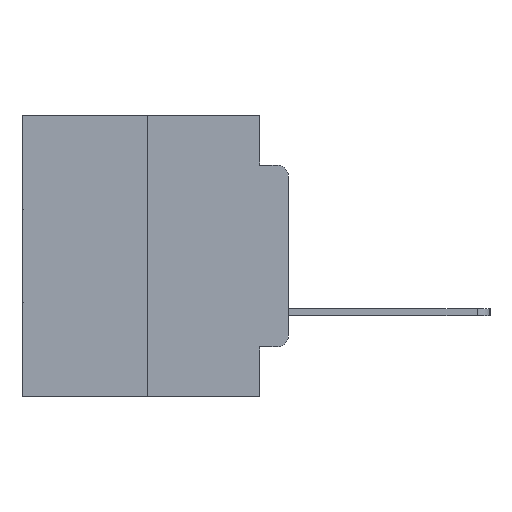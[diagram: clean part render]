
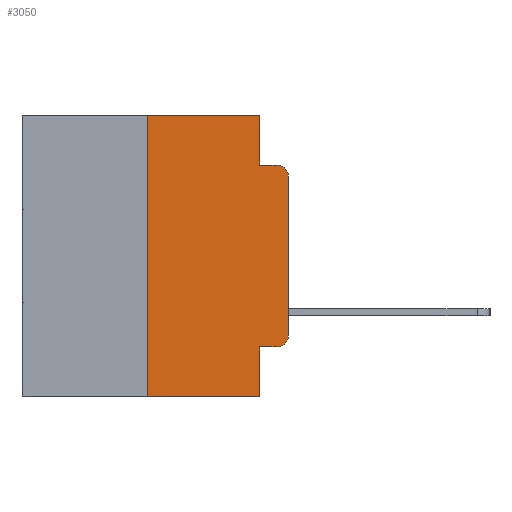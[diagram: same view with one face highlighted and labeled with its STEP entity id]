
A CAD part, left-side view. The second image highlights one B-rep face of the part: STEP entity #3050.
In plain terms, the highlighted planar face has unit normal (-1, 0, 0).
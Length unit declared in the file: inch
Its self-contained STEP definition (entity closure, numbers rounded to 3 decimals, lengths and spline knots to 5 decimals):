
#287 = LINE ( 'NONE', #20681, #16627 ) ;
#682 = VERTEX_POINT ( 'NONE', #21730 ) ;
#953 = VERTEX_POINT ( 'NONE', #15292 ) ;
#1065 = CARTESIAN_POINT ( 'NONE',  ( 0., 0.051, -0.0885 ) ) ;
#1193 = VECTOR ( 'NONE', #20912, 39.37008 ) ;
#1335 = VERTEX_POINT ( 'NONE', #1065 ) ;
#1770 = DIRECTION ( 'NONE',  ( -1., 0., 0. ) ) ;
#2549 = LINE ( 'NONE', #22921, #1193 ) ;
#3050 = ADVANCED_FACE ( 'NONE', ( #18681 ), #3953, .F. ) ;
#3126 = VERTEX_POINT ( 'NONE', #4517 ) ;
#3330 = ORIENTED_EDGE ( 'NONE', *, *, #9756, .F. ) ;
#3758 = CARTESIAN_POINT ( 'NONE',  ( 0., 0., -0.1085 ) ) ;
#3865 = CARTESIAN_POINT ( 'NONE',  ( 0., 0.473, -0.5 ) ) ;
#3953 = PLANE ( 'NONE',  #22412 ) ;
#4390 = VECTOR ( 'NONE', #15495, 39.37008 ) ;
#4517 = CARTESIAN_POINT ( 'NONE',  ( 0., 0.051, 0. ) ) ;
#4743 = CARTESIAN_POINT ( 'NONE',  ( 0., 0.051, -0.4115 ) ) ;
#4777 = AXIS2_PLACEMENT_3D ( 'NONE', #14542, #1770, #16639 ) ;
#5017 = CARTESIAN_POINT ( 'NONE',  ( 0., 0.051, -0.4115 ) ) ;
#5061 = CARTESIAN_POINT ( 'NONE',  ( 0., 0.051, 0. ) ) ;
#5077 = LINE ( 'NONE', #5017, #4390 ) ;
#5211 = VERTEX_POINT ( 'NONE', #20347 ) ;
#5696 = DIRECTION ( 'NONE',  ( 0., 0., 1. ) ) ;
#6668 = LINE ( 'NONE', #22225, #12323 ) ;
#6781 = CIRCLE ( 'NONE', #16351, 0.02 ) ;
#7011 = VERTEX_POINT ( 'NONE', #22452 ) ;
#7054 = EDGE_CURVE ( 'NONE', #9813, #682, #10407, .T. ) ;
#7096 = CARTESIAN_POINT ( 'NONE',  ( 0., 0.25, 0. ) ) ;
#7730 = ORIENTED_EDGE ( 'NONE', *, *, #14935, .T. ) ;
#7987 = EDGE_CURVE ( 'NONE', #26678, #3126, #14016, .T. ) ;
#8109 = CARTESIAN_POINT ( 'NONE',  ( 0., 0.473, 0. ) ) ;
#8330 = DIRECTION ( 'NONE',  ( 0., -1., 0. ) ) ;
#8448 = VECTOR ( 'NONE', #17324, 39.37008 ) ;
#8836 = VERTEX_POINT ( 'NONE', #9637 ) ;
#9637 = CARTESIAN_POINT ( 'NONE',  ( 0., 0.25, -0.5 ) ) ;
#9711 = VECTOR ( 'NONE', #12761, 39.37008 ) ;
#9756 = EDGE_CURVE ( 'NONE', #8836, #26678, #6668, .T. ) ;
#9813 = VERTEX_POINT ( 'NONE', #3758 ) ;
#9987 = EDGE_CURVE ( 'NONE', #23735, #7011, #2549, .T. ) ;
#10373 = LINE ( 'NONE', #14833, #9711 ) ;
#10398 = ORIENTED_EDGE ( 'NONE', *, *, #20171, .F. ) ;
#10407 = CIRCLE ( 'NONE', #4777, 0.02 ) ;
#10725 = EDGE_CURVE ( 'NONE', #3126, #1335, #20560, .T. ) ;
#11548 = DIRECTION ( 'NONE',  ( -1., 0., 0. ) ) ;
#12323 = VECTOR ( 'NONE', #5696, 39.37008 ) ;
#12624 = DIRECTION ( 'NONE',  ( 0., 0., -1. ) ) ;
#12761 = DIRECTION ( 'NONE',  ( 0., 0., 1. ) ) ;
#13661 = EDGE_CURVE ( 'NONE', #953, #5211, #6781, .T. ) ;
#14016 = LINE ( 'NONE', #15214, #8448 ) ;
#14495 = VECTOR ( 'NONE', #17643, 39.37008 ) ;
#14542 = CARTESIAN_POINT ( 'NONE',  ( 0., 0.02, -0.1085 ) ) ;
#14612 = ORIENTED_EDGE ( 'NONE', *, *, #7987, .F. ) ;
#14833 = CARTESIAN_POINT ( 'NONE',  ( 0., 0., 0. ) ) ;
#14935 = EDGE_CURVE ( 'NONE', #5211, #9813, #10373, .T. ) ;
#15214 = CARTESIAN_POINT ( 'NONE',  ( 0., 0.473, 0. ) ) ;
#15292 = CARTESIAN_POINT ( 'NONE',  ( 0., 0.02, -0.4115 ) ) ;
#15495 = DIRECTION ( 'NONE',  ( 0., -1., 0. ) ) ;
#15611 = ORIENTED_EDGE ( 'NONE', *, *, #13661, .T. ) ;
#16351 = AXIS2_PLACEMENT_3D ( 'NONE', #23712, #11548, #25697 ) ;
#16627 = VECTOR ( 'NONE', #8330, 39.37008 ) ;
#16639 = DIRECTION ( 'NONE',  ( 0., 0., -1. ) ) ;
#17220 = EDGE_CURVE ( 'NONE', #8836, #7011, #19909, .T. ) ;
#17324 = DIRECTION ( 'NONE',  ( 0., -1., 0. ) ) ;
#17643 = DIRECTION ( 'NONE',  ( 0., 0., -1. ) ) ;
#18681 = FACE_OUTER_BOUND ( 'NONE', #19276, .T. ) ;
#18788 = ORIENTED_EDGE ( 'NONE', *, *, #7054, .T. ) ;
#19276 = EDGE_LOOP ( 'NONE', ( #7730, #18788, #10398, #21920, #14612, #3330, #25946, #25743, #26275, #15611 ) ) ;
#19279 = VECTOR ( 'NONE', #20575, 39.37008 ) ;
#19909 = LINE ( 'NONE', #3865, #19279 ) ;
#20171 = EDGE_CURVE ( 'NONE', #1335, #682, #287, .T. ) ;
#20347 = CARTESIAN_POINT ( 'NONE',  ( 0., 0., -0.3915 ) ) ;
#20560 = LINE ( 'NONE', #5061, #14495 ) ;
#20575 = DIRECTION ( 'NONE',  ( 0., -1., 0. ) ) ;
#20681 = CARTESIAN_POINT ( 'NONE',  ( 0., 0.051, -0.0885 ) ) ;
#20912 = DIRECTION ( 'NONE',  ( 0., 0., -1. ) ) ;
#21682 = EDGE_CURVE ( 'NONE', #23735, #953, #5077, .T. ) ;
#21730 = CARTESIAN_POINT ( 'NONE',  ( 0., 0.02, -0.0885 ) ) ;
#21920 = ORIENTED_EDGE ( 'NONE', *, *, #10725, .F. ) ;
#22225 = CARTESIAN_POINT ( 'NONE',  ( 0., 0.25, 0. ) ) ;
#22412 = AXIS2_PLACEMENT_3D ( 'NONE', #8109, #24728, #12624 ) ;
#22452 = CARTESIAN_POINT ( 'NONE',  ( 0., 0.051, -0.5 ) ) ;
#22921 = CARTESIAN_POINT ( 'NONE',  ( 0., 0.051, 0. ) ) ;
#23712 = CARTESIAN_POINT ( 'NONE',  ( 0., 0.02, -0.3915 ) ) ;
#23735 = VERTEX_POINT ( 'NONE', #4743 ) ;
#24728 = DIRECTION ( 'NONE',  ( 1., 0., 0. ) ) ;
#25697 = DIRECTION ( 'NONE',  ( 0., 0., -1. ) ) ;
#25743 = ORIENTED_EDGE ( 'NONE', *, *, #9987, .F. ) ;
#25946 = ORIENTED_EDGE ( 'NONE', *, *, #17220, .T. ) ;
#26275 = ORIENTED_EDGE ( 'NONE', *, *, #21682, .T. ) ;
#26678 = VERTEX_POINT ( 'NONE', #7096 ) ;
